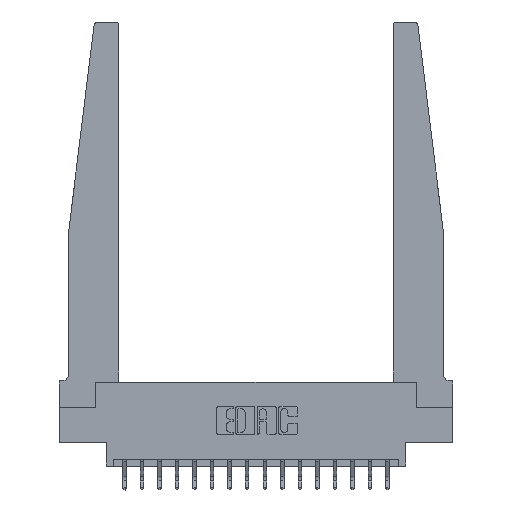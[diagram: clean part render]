
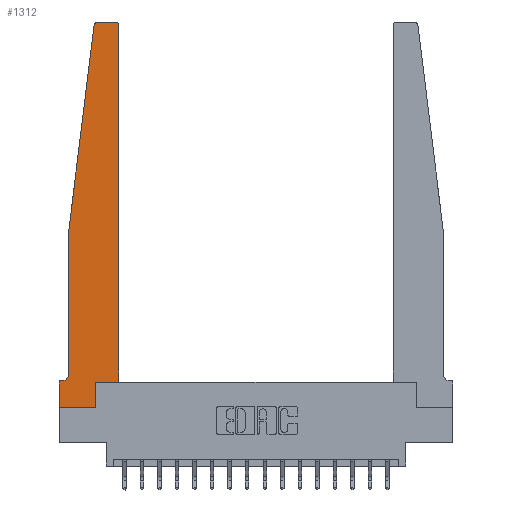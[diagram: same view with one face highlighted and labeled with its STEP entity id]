
A CAD part, top view. The second image highlights one B-rep face of the part: STEP entity #1312.
In plain terms, the highlighted planar face has unit normal (0, 0, 1).
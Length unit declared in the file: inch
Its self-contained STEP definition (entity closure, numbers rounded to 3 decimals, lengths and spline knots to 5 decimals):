
#41 = CARTESIAN_POINT ( 'NONE',  ( 0.395, 2.72, 0.37 ) ) ;
#481 = CARTESIAN_POINT ( 'NONE',  ( 0.065, 0.1875, 0.37 ) ) ;
#506 = EDGE_CURVE ( 'NONE', #18178, #6218, #16337, .T. ) ;
#513 = VECTOR ( 'NONE', #18215, 39.37008 ) ;
#989 = VECTOR ( 'NONE', #10398, 39.37008 ) ;
#1096 = CARTESIAN_POINT ( 'NONE',  ( 0.2605, 0.18, 0.37 ) ) ;
#1155 = VERTEX_POINT ( 'NONE', #17475 ) ;
#1185 = CARTESIAN_POINT ( 'NONE',  ( 0.425, 2.72, 0.37 ) ) ;
#1312 = ADVANCED_FACE ( 'NONE', ( #4903 ), #10436, .T. ) ;
#1334 = VERTEX_POINT ( 'NONE', #1597 ) ;
#1500 = DIRECTION ( 'NONE',  ( 1., 0., 0. ) ) ;
#1597 = CARTESIAN_POINT ( 'NONE',  ( 0.015, 0.1875, 0.37 ) ) ;
#2293 = EDGE_CURVE ( 'NONE', #1155, #4072, #11766, .T. ) ;
#2582 = VERTEX_POINT ( 'NONE', #2997 ) ;
#2818 = EDGE_LOOP ( 'NONE', ( #6144, #10160, #5570, #8147, #8620, #8163, #3354, #12442, #9597, #14088, #16922, #14726 ) ) ;
#2997 = CARTESIAN_POINT ( 'NONE',  ( 0.24675, 2.72367, 0.37 ) ) ;
#3046 = CARTESIAN_POINT ( 'NONE',  ( 0., 0.1875, 0.37 ) ) ;
#3109 = DIRECTION ( 'NONE',  ( 1., 0., 0. ) ) ;
#3354 = ORIENTED_EDGE ( 'NONE', *, *, #2293, .T. ) ;
#3387 = CARTESIAN_POINT ( 'NONE',  ( 0., 0., 0.37 ) ) ;
#3754 = EDGE_CURVE ( 'NONE', #9232, #1334, #16115, .T. ) ;
#4003 = DIRECTION ( 'NONE',  ( 0., 1., 0. ) ) ;
#4072 = VERTEX_POINT ( 'NONE', #3387 ) ;
#4095 = DIRECTION ( 'NONE',  ( 0., 1., 0. ) ) ;
#4192 = CARTESIAN_POINT ( 'NONE',  ( 0.2605, 0.18, 0.37 ) ) ;
#4402 = CARTESIAN_POINT ( 'NONE',  ( 0.425, 0.18, 0.37 ) ) ;
#4732 = CARTESIAN_POINT ( 'NONE',  ( 0.27653, 2.72, 0.37 ) ) ;
#4765 = VECTOR ( 'NONE', #11792, 39.37008 ) ;
#4903 = FACE_OUTER_BOUND ( 'NONE', #2818, .T. ) ;
#4949 = CARTESIAN_POINT ( 'NONE',  ( 0.25, 2.75, 0.37 ) ) ;
#5380 = DIRECTION ( 'NONE',  ( 0., -1., 0. ) ) ;
#5570 = ORIENTED_EDGE ( 'NONE', *, *, #7072, .T. ) ;
#5766 = CARTESIAN_POINT ( 'NONE',  ( 0.015, 0.2375, 0.37 ) ) ;
#5935 = VECTOR ( 'NONE', #15713, 39.37008 ) ;
#6144 = ORIENTED_EDGE ( 'NONE', *, *, #8462, .T. ) ;
#6202 = DIRECTION ( 'NONE',  ( 1., 0., 0. ) ) ;
#6218 = VERTEX_POINT ( 'NONE', #4192 ) ;
#6626 = VERTEX_POINT ( 'NONE', #11012 ) ;
#6859 = VERTEX_POINT ( 'NONE', #8596 ) ;
#7072 = EDGE_CURVE ( 'NONE', #2582, #6859, #13241, .T. ) ;
#7249 = DIRECTION ( 'NONE',  ( -1., 0., 0. ) ) ;
#7251 = CIRCLE ( 'NONE', #17947, 0.03 ) ;
#7853 = VECTOR ( 'NONE', #5380, 39.37008 ) ;
#8147 = ORIENTED_EDGE ( 'NONE', *, *, #13481, .T. ) ;
#8163 = ORIENTED_EDGE ( 'NONE', *, *, #18915, .T. ) ;
#8197 = EDGE_CURVE ( 'NONE', #14065, #8576, #16464, .T. ) ;
#8462 = EDGE_CURVE ( 'NONE', #8576, #6626, #12288, .T. ) ;
#8565 = CARTESIAN_POINT ( 'NONE',  ( 0.2605, 0., 0.37 ) ) ;
#8576 = VERTEX_POINT ( 'NONE', #12546 ) ;
#8596 = CARTESIAN_POINT ( 'NONE',  ( 0.065, 1.25, 0.37 ) ) ;
#8620 = ORIENTED_EDGE ( 'NONE', *, *, #3754, .T. ) ;
#9232 = VERTEX_POINT ( 'NONE', #18697 ) ;
#9597 = ORIENTED_EDGE ( 'NONE', *, *, #506, .T. ) ;
#9852 = LINE ( 'NONE', #17182, #5935 ) ;
#9968 = CARTESIAN_POINT ( 'NONE',  ( 0.425, 0.18, 0.37 ) ) ;
#10147 = VERTEX_POINT ( 'NONE', #4402 ) ;
#10160 = ORIENTED_EDGE ( 'NONE', *, *, #15114, .T. ) ;
#10310 = CARTESIAN_POINT ( 'NONE',  ( 0.065, 1.25, 0.37 ) ) ;
#10351 = DIRECTION ( 'NONE',  ( 0., 0., 1. ) ) ;
#10398 = DIRECTION ( 'NONE',  ( -0.122, -0.992, 0. ) ) ;
#10436 = PLANE ( 'NONE',  #12789 ) ;
#10547 = VECTOR ( 'NONE', #13559, 39.37008 ) ;
#10808 = DIRECTION ( 'NONE',  ( -1., 0., 0. ) ) ;
#11012 = CARTESIAN_POINT ( 'NONE',  ( 0.27653, 2.75, 0.37 ) ) ;
#11074 = LINE ( 'NONE', #481, #17981 ) ;
#11619 = EDGE_CURVE ( 'NONE', #4072, #18178, #18391, .T. ) ;
#11766 = LINE ( 'NONE', #17189, #7853 ) ;
#11792 = DIRECTION ( 'NONE',  ( 0., -1., 0. ) ) ;
#11926 = DIRECTION ( 'NONE',  ( 0., 0., 1. ) ) ;
#12058 = CARTESIAN_POINT ( 'NONE',  ( 0., 0., 0.37 ) ) ;
#12119 = EDGE_CURVE ( 'NONE', #10147, #14065, #18370, .T. ) ;
#12288 = LINE ( 'NONE', #4949, #513 ) ;
#12409 = VECTOR ( 'NONE', #4095, 39.37008 ) ;
#12442 = ORIENTED_EDGE ( 'NONE', *, *, #11619, .T. ) ;
#12546 = CARTESIAN_POINT ( 'NONE',  ( 0.395, 2.75, 0.37 ) ) ;
#12593 = LINE ( 'NONE', #10310, #4765 ) ;
#12685 = EDGE_CURVE ( 'NONE', #6218, #10147, #9852, .T. ) ;
#12789 = AXIS2_PLACEMENT_3D ( 'NONE', #3046, #11926, #3109 ) ;
#13180 = AXIS2_PLACEMENT_3D ( 'NONE', #41, #10351, #1500 ) ;
#13241 = LINE ( 'NONE', #13443, #989 ) ;
#13443 = CARTESIAN_POINT ( 'NONE',  ( 0.065, 1.25, 0.37 ) ) ;
#13481 = EDGE_CURVE ( 'NONE', #6859, #9232, #12593, .T. ) ;
#13559 = DIRECTION ( 'NONE',  ( 1., 0., 0. ) ) ;
#14018 = VECTOR ( 'NONE', #4003, 39.37008 ) ;
#14065 = VERTEX_POINT ( 'NONE', #1185 ) ;
#14088 = ORIENTED_EDGE ( 'NONE', *, *, #12685, .T. ) ;
#14726 = ORIENTED_EDGE ( 'NONE', *, *, #8197, .T. ) ;
#15052 = DIRECTION ( 'NONE',  ( 0., 0., 1. ) ) ;
#15114 = EDGE_CURVE ( 'NONE', #6626, #2582, #7251, .T. ) ;
#15192 = AXIS2_PLACEMENT_3D ( 'NONE', #5766, #16099, #7249 ) ;
#15713 = DIRECTION ( 'NONE',  ( 1., 0., 0. ) ) ;
#16099 = DIRECTION ( 'NONE',  ( 0., 0., -1. ) ) ;
#16115 = CIRCLE ( 'NONE', #15192, 0.05 ) ;
#16337 = LINE ( 'NONE', #1096, #12409 ) ;
#16464 = CIRCLE ( 'NONE', #13180, 0.03 ) ;
#16922 = ORIENTED_EDGE ( 'NONE', *, *, #12119, .T. ) ;
#17182 = CARTESIAN_POINT ( 'NONE',  ( 0.425, 0.18, 0.37 ) ) ;
#17189 = CARTESIAN_POINT ( 'NONE',  ( 0., 0., 0.37 ) ) ;
#17475 = CARTESIAN_POINT ( 'NONE',  ( 0., 0.1875, 0.37 ) ) ;
#17947 = AXIS2_PLACEMENT_3D ( 'NONE', #4732, #15052, #6202 ) ;
#17981 = VECTOR ( 'NONE', #10808, 39.37008 ) ;
#18178 = VERTEX_POINT ( 'NONE', #8565 ) ;
#18215 = DIRECTION ( 'NONE',  ( -1., 0., 0. ) ) ;
#18370 = LINE ( 'NONE', #9968, #14018 ) ;
#18391 = LINE ( 'NONE', #12058, #10547 ) ;
#18697 = CARTESIAN_POINT ( 'NONE',  ( 0.065, 0.2375, 0.37 ) ) ;
#18915 = EDGE_CURVE ( 'NONE', #1334, #1155, #11074, .T. ) ;
